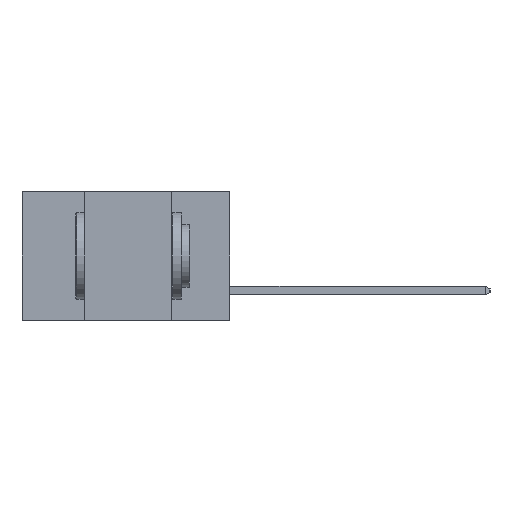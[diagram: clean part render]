
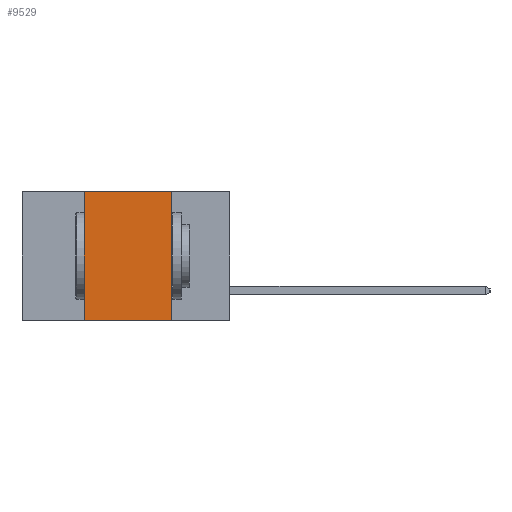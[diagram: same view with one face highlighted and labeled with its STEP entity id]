
A CAD part, left-side view. The second image highlights one B-rep face of the part: STEP entity #9529.
In plain terms, the highlighted planar face has unit normal (-1, 0, 0).
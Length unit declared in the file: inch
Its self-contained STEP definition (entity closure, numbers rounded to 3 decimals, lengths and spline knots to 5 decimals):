
#141 = CARTESIAN_POINT ( 'NONE',  ( 0., 0.42, -0.37 ) ) ;
#1272 = CARTESIAN_POINT ( 'NONE',  ( 0., 0.6, 0. ) ) ;
#1366 = VECTOR ( 'NONE', #7791, 39.37008 ) ;
#1470 = DIRECTION ( 'NONE',  ( 0., -1., 0. ) ) ;
#1695 = CARTESIAN_POINT ( 'NONE',  ( 0., 0.17, 0. ) ) ;
#1756 = ORIENTED_EDGE ( 'NONE', *, *, #3057, .F. ) ;
#3057 = EDGE_CURVE ( 'NONE', #19325, #4855, #7918, .T. ) ;
#3306 = LINE ( 'NONE', #10211, #19678 ) ;
#4197 = VECTOR ( 'NONE', #1470, 39.37008 ) ;
#4855 = VERTEX_POINT ( 'NONE', #1695 ) ;
#5830 = AXIS2_PLACEMENT_3D ( 'NONE', #14459, #14452, #14428 ) ;
#6133 = CARTESIAN_POINT ( 'NONE',  ( 0., 0.17, -0.37 ) ) ;
#6967 = ORIENTED_EDGE ( 'NONE', *, *, #13092, .T. ) ;
#7294 = EDGE_CURVE ( 'NONE', #4855, #8718, #12042, .T. ) ;
#7772 = VECTOR ( 'NONE', #8119, 39.37008 ) ;
#7791 = DIRECTION ( 'NONE',  ( 0., 0., 1. ) ) ;
#7918 = LINE ( 'NONE', #1272, #4197 ) ;
#8119 = DIRECTION ( 'NONE',  ( 0., 0., -1. ) ) ;
#8718 = VERTEX_POINT ( 'NONE', #6133 ) ;
#8776 = CARTESIAN_POINT ( 'NONE',  ( 0., 0.17, -0.37 ) ) ;
#9529 = ADVANCED_FACE ( 'NONE', ( #11447 ), #14547, .F. ) ;
#10211 = CARTESIAN_POINT ( 'NONE',  ( 0., 0.6, -0.37 ) ) ;
#10493 = DIRECTION ( 'NONE',  ( 0., -1., 0. ) ) ;
#11447 = FACE_OUTER_BOUND ( 'NONE', #14801, .T. ) ;
#12042 = LINE ( 'NONE', #8776, #7772 ) ;
#12349 = CARTESIAN_POINT ( 'NONE',  ( 0., 0.42, 0. ) ) ;
#13092 = EDGE_CURVE ( 'NONE', #19922, #8718, #3306, .T. ) ;
#14428 = DIRECTION ( 'NONE',  ( 0., 0., -1. ) ) ;
#14452 = DIRECTION ( 'NONE',  ( 1., 0., 0. ) ) ;
#14459 = CARTESIAN_POINT ( 'NONE',  ( 0., 0.6, 0. ) ) ;
#14547 = PLANE ( 'NONE',  #5830 ) ;
#14801 = EDGE_LOOP ( 'NONE', ( #18186, #1756, #19166, #6967 ) ) ;
#17437 = CARTESIAN_POINT ( 'NONE',  ( 0., 0.42, -0.37 ) ) ;
#18186 = ORIENTED_EDGE ( 'NONE', *, *, #7294, .F. ) ;
#18295 = LINE ( 'NONE', #17437, #1366 ) ;
#19166 = ORIENTED_EDGE ( 'NONE', *, *, #19437, .F. ) ;
#19325 = VERTEX_POINT ( 'NONE', #12349 ) ;
#19437 = EDGE_CURVE ( 'NONE', #19922, #19325, #18295, .T. ) ;
#19678 = VECTOR ( 'NONE', #10493, 39.37008 ) ;
#19922 = VERTEX_POINT ( 'NONE', #141 ) ;
